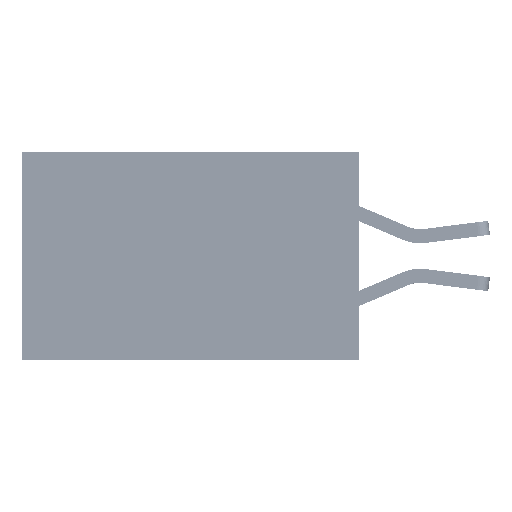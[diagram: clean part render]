
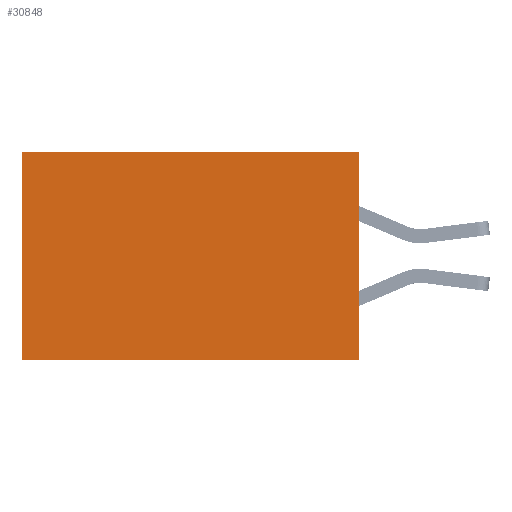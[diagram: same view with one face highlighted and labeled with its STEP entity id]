
A CAD part, left-side view. The second image highlights one B-rep face of the part: STEP entity #30848.
In plain terms, the highlighted planar face has unit normal (-1, 0, 0).
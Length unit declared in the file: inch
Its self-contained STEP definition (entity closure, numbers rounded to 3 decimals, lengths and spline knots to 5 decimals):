
#192 = VECTOR ( 'NONE', #43903, 39.37008 ) ;
#404 = EDGE_LOOP ( 'NONE', ( #37653, #42528, #43148, #14770 ) ) ;
#473 = CARTESIAN_POINT ( 'NONE',  ( 0.2875, 0., 0. ) ) ;
#1903 = CARTESIAN_POINT ( 'NONE',  ( 0.2875, 0., -0.37 ) ) ;
#2496 = VERTEX_POINT ( 'NONE', #42529 ) ;
#4718 = DIRECTION ( 'NONE',  ( 0., 1., 0. ) ) ;
#6728 = CARTESIAN_POINT ( 'NONE',  ( 0.2875, 0., 0. ) ) ;
#7598 = VECTOR ( 'NONE', #14991, 39.37008 ) ;
#11705 = LINE ( 'NONE', #41349, #20741 ) ;
#14710 = DIRECTION ( 'NONE',  ( 0., 0., -1. ) ) ;
#14770 = ORIENTED_EDGE ( 'NONE', *, *, #16130, .T. ) ;
#14991 = DIRECTION ( 'NONE',  ( 0., 0., -1. ) ) ;
#15103 = LINE ( 'NONE', #30806, #192 ) ;
#15804 = VERTEX_POINT ( 'NONE', #28597 ) ;
#16130 = EDGE_CURVE ( 'NONE', #35480, #2496, #15103, .T. ) ;
#18544 = EDGE_CURVE ( 'NONE', #35480, #15804, #25743, .T. ) ;
#20741 = VECTOR ( 'NONE', #14710, 39.37008 ) ;
#21198 = DIRECTION ( 'NONE',  ( 0., 0., -1. ) ) ;
#22619 = CARTESIAN_POINT ( 'NONE',  ( 0.2875, 0.6, -0.37 ) ) ;
#23582 = EDGE_CURVE ( 'NONE', #15804, #24128, #42549, .T. ) ;
#24128 = VERTEX_POINT ( 'NONE', #22619 ) ;
#25171 = AXIS2_PLACEMENT_3D ( 'NONE', #473, #38251, #21198 ) ;
#25743 = LINE ( 'NONE', #34923, #7598 ) ;
#28597 = CARTESIAN_POINT ( 'NONE',  ( 0.2875, 0., -0.37 ) ) ;
#30806 = CARTESIAN_POINT ( 'NONE',  ( 0.2875, 0., 0. ) ) ;
#30848 = ADVANCED_FACE ( 'NONE', ( #36004 ), #41690, .F. ) ;
#34251 = EDGE_CURVE ( 'NONE', #2496, #24128, #11705, .T. ) ;
#34923 = CARTESIAN_POINT ( 'NONE',  ( 0.2875, 0., 0. ) ) ;
#35480 = VERTEX_POINT ( 'NONE', #6728 ) ;
#36004 = FACE_OUTER_BOUND ( 'NONE', #404, .T. ) ;
#37653 = ORIENTED_EDGE ( 'NONE', *, *, #34251, .T. ) ;
#38251 = DIRECTION ( 'NONE',  ( 1., 0., 0. ) ) ;
#38839 = VECTOR ( 'NONE', #4718, 39.37008 ) ;
#41349 = CARTESIAN_POINT ( 'NONE',  ( 0.2875, 0.6, 0. ) ) ;
#41690 = PLANE ( 'NONE',  #25171 ) ;
#42528 = ORIENTED_EDGE ( 'NONE', *, *, #23582, .F. ) ;
#42529 = CARTESIAN_POINT ( 'NONE',  ( 0.2875, 0.6, 0. ) ) ;
#42549 = LINE ( 'NONE', #1903, #38839 ) ;
#43148 = ORIENTED_EDGE ( 'NONE', *, *, #18544, .F. ) ;
#43903 = DIRECTION ( 'NONE',  ( 0., 1., 0. ) ) ;
